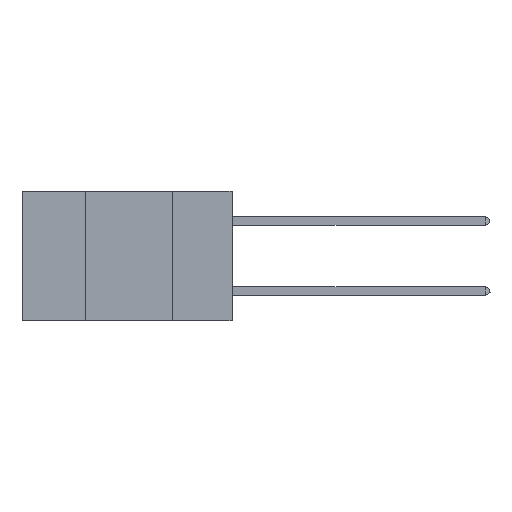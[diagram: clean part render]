
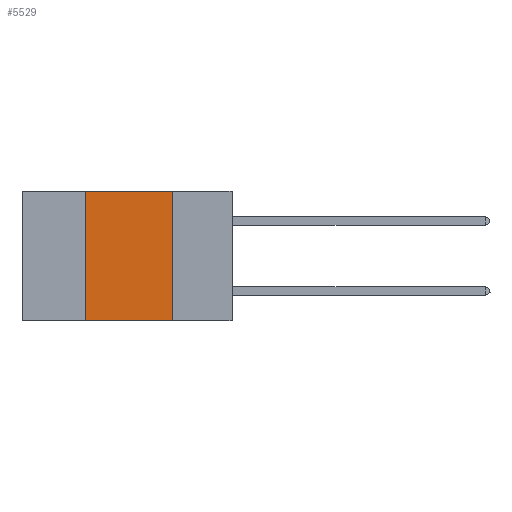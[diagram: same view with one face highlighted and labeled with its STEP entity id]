
A CAD part, left-side view. The second image highlights one B-rep face of the part: STEP entity #5529.
In plain terms, the highlighted planar face has unit normal (-1, 0, 0).
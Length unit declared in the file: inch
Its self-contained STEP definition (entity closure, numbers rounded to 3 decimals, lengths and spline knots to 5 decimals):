
#340 = DIRECTION ( 'NONE',  ( 0., 0., -1. ) ) ;
#404 = ORIENTED_EDGE ( 'NONE', *, *, #3274, .F. ) ;
#1058 = LINE ( 'NONE', #13151, #9157 ) ;
#2160 = DIRECTION ( 'NONE',  ( 0., 0., 1. ) ) ;
#2993 = CARTESIAN_POINT ( 'NONE',  ( 0., 0.42, 0. ) ) ;
#3133 = EDGE_LOOP ( 'NONE', ( #404, #7840, #26241, #3577 ) ) ;
#3274 = EDGE_CURVE ( 'NONE', #3872, #21575, #22530, .T. ) ;
#3577 = ORIENTED_EDGE ( 'NONE', *, *, #8958, .T. ) ;
#3843 = AXIS2_PLACEMENT_3D ( 'NONE', #4407, #21194, #340 ) ;
#3872 = VERTEX_POINT ( 'NONE', #16535 ) ;
#4407 = CARTESIAN_POINT ( 'NONE',  ( 0., 0.6, 0. ) ) ;
#5529 = ADVANCED_FACE ( 'NONE', ( #12935 ), #10687, .F. ) ;
#6504 = CARTESIAN_POINT ( 'NONE',  ( 0., 0.42, 0. ) ) ;
#7110 = DIRECTION ( 'NONE',  ( 0., 0., -1. ) ) ;
#7132 = EDGE_CURVE ( 'NONE', #14168, #3872, #23317, .T. ) ;
#7653 = LINE ( 'NONE', #6504, #15899 ) ;
#7840 = ORIENTED_EDGE ( 'NONE', *, *, #7132, .F. ) ;
#8958 = EDGE_CURVE ( 'NONE', #11370, #21575, #1058, .T. ) ;
#9157 = VECTOR ( 'NONE', #25421, 39.37008 ) ;
#10687 = PLANE ( 'NONE',  #3843 ) ;
#11370 = VERTEX_POINT ( 'NONE', #21723 ) ;
#11771 = DIRECTION ( 'NONE',  ( 0., -1., 0. ) ) ;
#12935 = FACE_OUTER_BOUND ( 'NONE', #3133, .T. ) ;
#13151 = CARTESIAN_POINT ( 'NONE',  ( 0., 0.6, -0.37 ) ) ;
#14168 = VERTEX_POINT ( 'NONE', #2993 ) ;
#14472 = EDGE_CURVE ( 'NONE', #11370, #14168, #7653, .T. ) ;
#15899 = VECTOR ( 'NONE', #2160, 39.37008 ) ;
#16535 = CARTESIAN_POINT ( 'NONE',  ( 0., 0.17, 0. ) ) ;
#16653 = VECTOR ( 'NONE', #7110, 39.37008 ) ;
#19735 = VECTOR ( 'NONE', #11771, 39.37008 ) ;
#21194 = DIRECTION ( 'NONE',  ( 1., 0., 0. ) ) ;
#21575 = VERTEX_POINT ( 'NONE', #23051 ) ;
#21723 = CARTESIAN_POINT ( 'NONE',  ( 0., 0.42, -0.37 ) ) ;
#22530 = LINE ( 'NONE', #25900, #16653 ) ;
#23051 = CARTESIAN_POINT ( 'NONE',  ( 0., 0.17, -0.37 ) ) ;
#23317 = LINE ( 'NONE', #26611, #19735 ) ;
#25421 = DIRECTION ( 'NONE',  ( 0., -1., 0. ) ) ;
#25900 = CARTESIAN_POINT ( 'NONE',  ( 0., 0.17, 0. ) ) ;
#26241 = ORIENTED_EDGE ( 'NONE', *, *, #14472, .F. ) ;
#26611 = CARTESIAN_POINT ( 'NONE',  ( 0., 0.6, 0. ) ) ;
